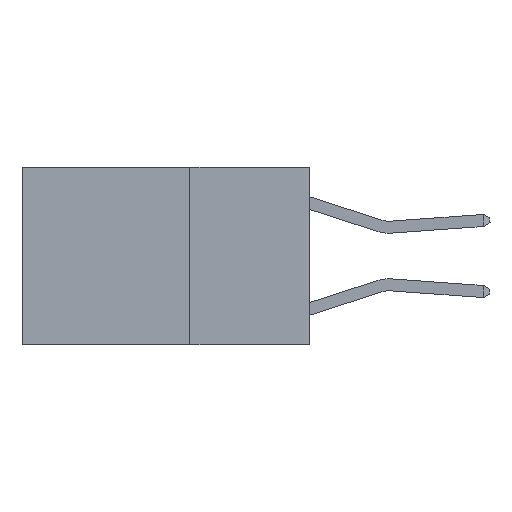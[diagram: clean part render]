
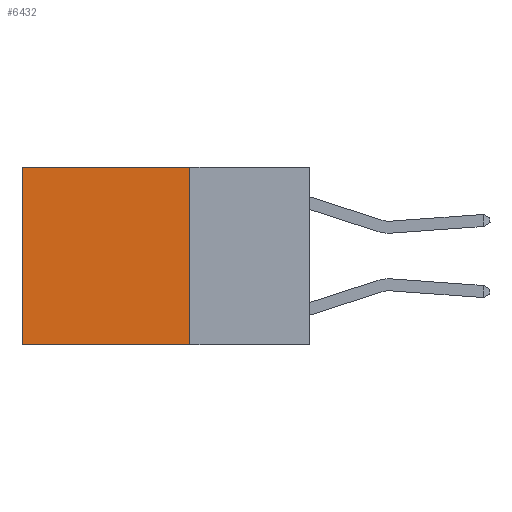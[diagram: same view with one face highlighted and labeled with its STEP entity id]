
A CAD part, left-side view. The second image highlights one B-rep face of the part: STEP entity #6432.
In plain terms, the highlighted planar face has unit normal (-1, 0, 0).
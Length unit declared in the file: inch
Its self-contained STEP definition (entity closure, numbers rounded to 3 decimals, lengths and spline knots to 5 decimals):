
#100 = EDGE_CURVE ( 'NONE', #1146, #2328, #10273, .T. ) ;
#133 = VECTOR ( 'NONE', #12704, 39.37008 ) ;
#655 = EDGE_LOOP ( 'NONE', ( #5088, #6281, #4812, #5115 ) ) ;
#827 = LINE ( 'NONE', #8446, #9081 ) ;
#1146 = VERTEX_POINT ( 'NONE', #2882 ) ;
#1838 = DIRECTION ( 'NONE',  ( 1., 0., 0. ) ) ;
#1890 = VECTOR ( 'NONE', #11728, 39.37008 ) ;
#1962 = FACE_OUTER_BOUND ( 'NONE', #655, .T. ) ;
#2149 = DIRECTION ( 'NONE',  ( 0., 1., 0. ) ) ;
#2328 = VERTEX_POINT ( 'NONE', #9958 ) ;
#2882 = CARTESIAN_POINT ( 'NONE',  ( 0.2625, 0.25, 0. ) ) ;
#3002 = LINE ( 'NONE', #10598, #133 ) ;
#3105 = VERTEX_POINT ( 'NONE', #7920 ) ;
#3183 = CARTESIAN_POINT ( 'NONE',  ( 0.2625, 0.25, -0.37 ) ) ;
#3657 = AXIS2_PLACEMENT_3D ( 'NONE', #11258, #1838, #9211 ) ;
#4595 = VERTEX_POINT ( 'NONE', #6286 ) ;
#4677 = CARTESIAN_POINT ( 'NONE',  ( 0.2625, 0.25, 0. ) ) ;
#4812 = ORIENTED_EDGE ( 'NONE', *, *, #100, .F. ) ;
#5088 = ORIENTED_EDGE ( 'NONE', *, *, #13510, .T. ) ;
#5115 = ORIENTED_EDGE ( 'NONE', *, *, #13454, .T. ) ;
#5245 = LINE ( 'NONE', #3183, #8013 ) ;
#6281 = ORIENTED_EDGE ( 'NONE', *, *, #10828, .F. ) ;
#6286 = CARTESIAN_POINT ( 'NONE',  ( 0.2625, 0.6, 0. ) ) ;
#6432 = ADVANCED_FACE ( 'NONE', ( #1962 ), #12309, .F. ) ;
#7920 = CARTESIAN_POINT ( 'NONE',  ( 0.2625, 0.6, -0.37 ) ) ;
#8013 = VECTOR ( 'NONE', #11577, 39.37008 ) ;
#8446 = CARTESIAN_POINT ( 'NONE',  ( 0.2625, 0.25, 0. ) ) ;
#9081 = VECTOR ( 'NONE', #2149, 39.37008 ) ;
#9211 = DIRECTION ( 'NONE',  ( 0., 0., -1. ) ) ;
#9958 = CARTESIAN_POINT ( 'NONE',  ( 0.2625, 0.25, -0.37 ) ) ;
#10273 = LINE ( 'NONE', #4677, #1890 ) ;
#10598 = CARTESIAN_POINT ( 'NONE',  ( 0.2625, 0.6, 0. ) ) ;
#10828 = EDGE_CURVE ( 'NONE', #2328, #3105, #5245, .T. ) ;
#11258 = CARTESIAN_POINT ( 'NONE',  ( 0.2625, 0.25, 0. ) ) ;
#11577 = DIRECTION ( 'NONE',  ( 0., 1., 0. ) ) ;
#11728 = DIRECTION ( 'NONE',  ( 0., 0., -1. ) ) ;
#12309 = PLANE ( 'NONE',  #3657 ) ;
#12704 = DIRECTION ( 'NONE',  ( 0., 0., -1. ) ) ;
#13454 = EDGE_CURVE ( 'NONE', #1146, #4595, #827, .T. ) ;
#13510 = EDGE_CURVE ( 'NONE', #4595, #3105, #3002, .T. ) ;
